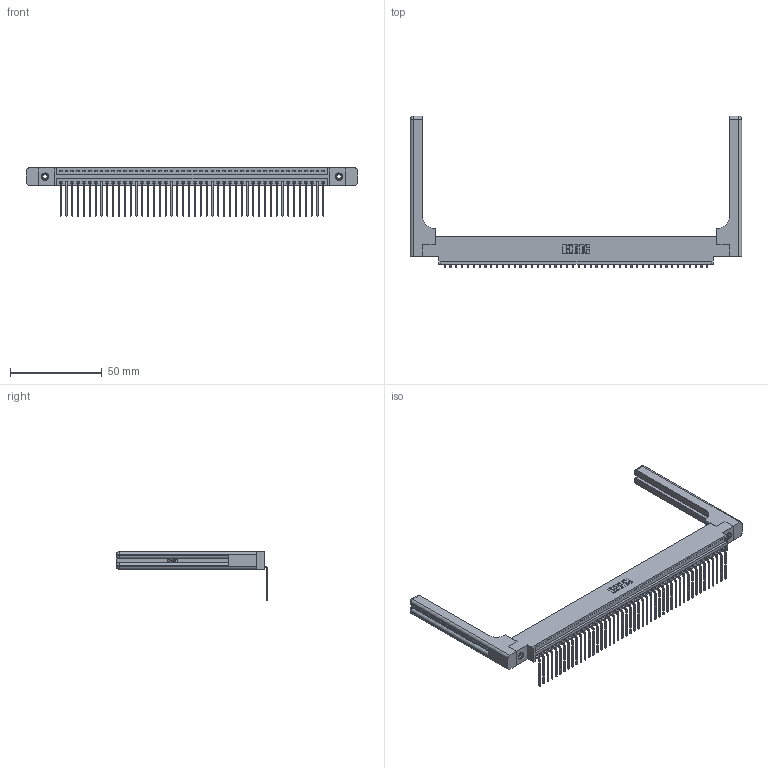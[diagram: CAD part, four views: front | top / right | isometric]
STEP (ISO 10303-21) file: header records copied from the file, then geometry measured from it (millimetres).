
FILE_DESCRIPTION (( 'STEP AP203' ), '1' );
FILE_NAME ('396-046-559-658.STEP', '2019-10-31T23:24:10', ( '' ), ( '' ), 'SwSTEP 2.0', 'SolidWorks 2016', '' );
FILE_SCHEMA (( 'CONFIG_CONTROL_DESIGN' ));
Length unit declared in the file: inch
Products named in the file (5): 346 Part_0.170 Offset - 0.156 Dia-TH; 345-292-001_558 559 Tail - 1; 345-250-001_345-250-001-102; 346-220-058_345-220-058; 396-046-559-658
Assembly tree (51 placements, depth 2):
  396-046-559-658
    346 Part_0.170 Offset - 0.156 Dia-TH
    345-292-001_558 559 Tail - 1  x46
    345-250-001_345-250-001-102  x2
    346-220-058_345-220-058  x2
Bounding box: 180.11 x 82.36 x 26.16 mm (x, y, z)
Volume: 24785.2 mm3; surface area: 27868.7 mm2
Topology: 51 solids, 51 shells, 3142 faces, 9379 edges, 6170 vertices
Faces by surface type: plane 2160, cylinder 922, bspline 36, cone 12, sphere 8, torus 4
Entity records: 33408 total; most frequent: CARTESIAN_POINT 6707, ORIENTED_EDGE 5484, DIRECTION 4842, EDGE_CURVE 2742, VECTOR 2334, LINE 2334, VERTEX_POINT 1818, AXIS2_PLACEMENT_3D 1254
